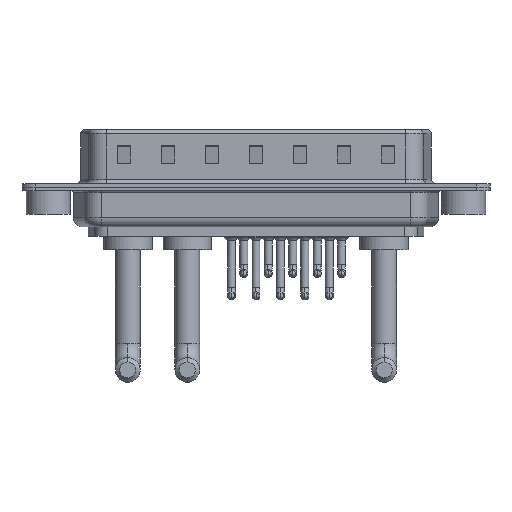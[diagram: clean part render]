
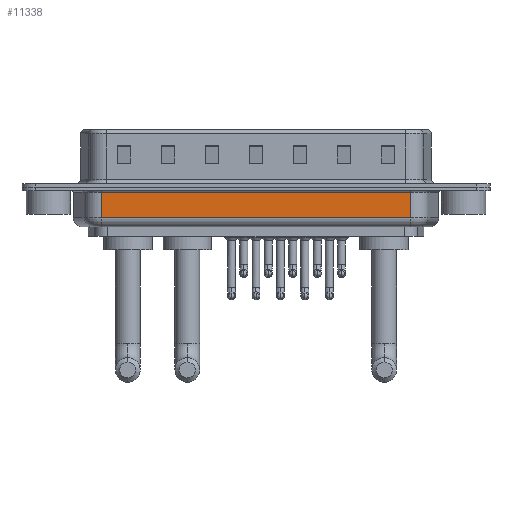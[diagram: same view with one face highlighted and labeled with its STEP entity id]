
A CAD part, front view. The second image highlights one B-rep face of the part: STEP entity #11338.
In plain terms, the highlighted planar face has unit normal (0, -1, 0).
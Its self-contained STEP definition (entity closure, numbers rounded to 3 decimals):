
#452 = EDGE_LOOP ( 'NONE', ( #22604, #16857, #4158, #594 ) ) ;
#594 = ORIENTED_EDGE ( 'NONE', *, *, #11389, .T. ) ;
#1144 = VECTOR ( 'NONE', #13634, 1000. ) ;
#1659 = CARTESIAN_POINT ( 'NONE',  ( 6.006, -5.35, -4.5 ) ) ;
#2848 = AXIS2_PLACEMENT_3D ( 'NONE', #15403, #11931, #13482 ) ;
#3226 = LINE ( 'NONE', #15744, #9883 ) ;
#3398 = EDGE_CURVE ( 'NONE', #19763, #23599, #6714, .T. ) ;
#3472 = VERTEX_POINT ( 'NONE', #8268 ) ;
#4158 = ORIENTED_EDGE ( 'NONE', *, *, #3398, .T. ) ;
#4802 = CARTESIAN_POINT ( 'NONE',  ( 41.044, -5.35, -4.5 ) ) ;
#6179 = EDGE_CURVE ( 'NONE', #22178, #19763, #12354, .T. ) ;
#6714 = LINE ( 'NONE', #4802, #1144 ) ;
#8002 = FACE_OUTER_BOUND ( 'NONE', #452, .T. ) ;
#8268 = CARTESIAN_POINT ( 'NONE',  ( 6.006, -5.35, -0.65 ) ) ;
#9883 = VECTOR ( 'NONE', #17889, 1000. ) ;
#10321 = DIRECTION ( 'NONE',  ( 1., 0., 0. ) ) ;
#10391 = VECTOR ( 'NONE', #10321, 1000. ) ;
#10605 = EDGE_CURVE ( 'NONE', #22178, #3472, #21724, .T. ) ;
#11338 = ADVANCED_FACE ( 'NONE', ( #8002 ), #11698, .F. ) ;
#11389 = EDGE_CURVE ( 'NONE', #23599, #3472, #3226, .T. ) ;
#11698 = PLANE ( 'NONE',  #2848 ) ;
#11931 = DIRECTION ( 'NONE',  ( 0., 1., 0. ) ) ;
#12354 = LINE ( 'NONE', #17624, #10391 ) ;
#12934 = CARTESIAN_POINT ( 'NONE',  ( 41.044, -5.35, -0.65 ) ) ;
#13482 = DIRECTION ( 'NONE',  ( 0., 0., 1. ) ) ;
#13634 = DIRECTION ( 'NONE',  ( 0., 0., 1. ) ) ;
#15403 = CARTESIAN_POINT ( 'NONE',  ( 6.006, -5.35, -4.5 ) ) ;
#15744 = CARTESIAN_POINT ( 'NONE',  ( 6.006, -5.35, -0.65 ) ) ;
#16438 = DIRECTION ( 'NONE',  ( 0., 0., 1. ) ) ;
#16857 = ORIENTED_EDGE ( 'NONE', *, *, #6179, .T. ) ;
#17624 = CARTESIAN_POINT ( 'NONE',  ( 6.006, -5.35, -3.5 ) ) ;
#17889 = DIRECTION ( 'NONE',  ( -1., 0., 0. ) ) ;
#19287 = CARTESIAN_POINT ( 'NONE',  ( 6.006, -5.35, -3.5 ) ) ;
#19763 = VERTEX_POINT ( 'NONE', #21880 ) ;
#21724 = LINE ( 'NONE', #1659, #23347 ) ;
#21880 = CARTESIAN_POINT ( 'NONE',  ( 41.044, -5.35, -3.5 ) ) ;
#22178 = VERTEX_POINT ( 'NONE', #19287 ) ;
#22604 = ORIENTED_EDGE ( 'NONE', *, *, #10605, .F. ) ;
#23347 = VECTOR ( 'NONE', #16438, 1000. ) ;
#23599 = VERTEX_POINT ( 'NONE', #12934 ) ;
